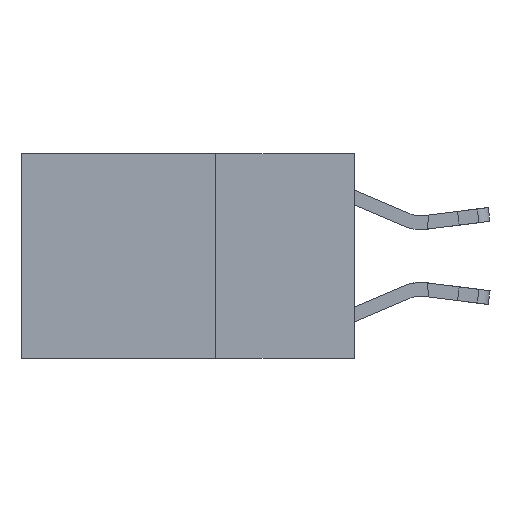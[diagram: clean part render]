
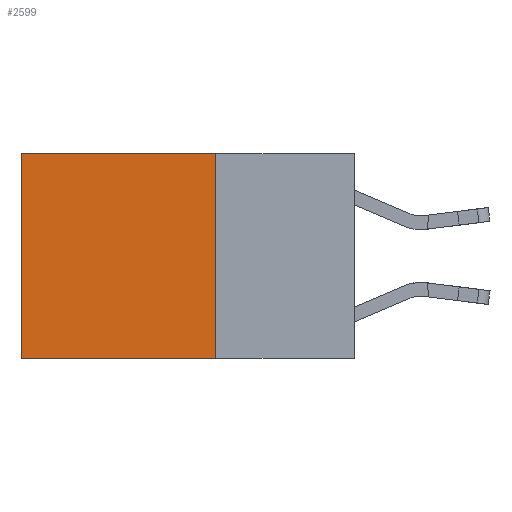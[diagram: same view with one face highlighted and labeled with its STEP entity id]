
A CAD part, left-side view. The second image highlights one B-rep face of the part: STEP entity #2599.
In plain terms, the highlighted planar face has unit normal (-1, 0, 0).
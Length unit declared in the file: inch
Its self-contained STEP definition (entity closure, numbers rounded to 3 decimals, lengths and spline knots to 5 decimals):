
#435 = VECTOR ( 'NONE', #5245, 39.37008 ) ;
#754 = LINE ( 'NONE', #13047, #18371 ) ;
#1513 = LINE ( 'NONE', #2937, #5573 ) ;
#1742 = DIRECTION ( 'NONE',  ( 0., 1., 0. ) ) ;
#2599 = ADVANCED_FACE ( 'NONE', ( #16636 ), #10279, .F. ) ;
#2937 = CARTESIAN_POINT ( 'NONE',  ( 0.2625, 0.25, 0. ) ) ;
#3076 = VERTEX_POINT ( 'NONE', #11743 ) ;
#3547 = ORIENTED_EDGE ( 'NONE', *, *, #13898, .T. ) ;
#5078 = VERTEX_POINT ( 'NONE', #19584 ) ;
#5245 = DIRECTION ( 'NONE',  ( 0., 0., -1. ) ) ;
#5573 = VECTOR ( 'NONE', #1742, 39.37008 ) ;
#5997 = ORIENTED_EDGE ( 'NONE', *, *, #12808, .F. ) ;
#6161 = EDGE_CURVE ( 'NONE', #3076, #11448, #14962, .T. ) ;
#6278 = AXIS2_PLACEMENT_3D ( 'NONE', #13685, #18794, #8661 ) ;
#7258 = ORIENTED_EDGE ( 'NONE', *, *, #6161, .F. ) ;
#7302 = EDGE_LOOP ( 'NONE', ( #21261, #7258, #5997, #3547 ) ) ;
#8661 = DIRECTION ( 'NONE',  ( 0., 0., -1. ) ) ;
#9458 = EDGE_CURVE ( 'NONE', #12452, #11448, #13536, .T. ) ;
#10279 = PLANE ( 'NONE',  #6278 ) ;
#10459 = VECTOR ( 'NONE', #15461, 39.37008 ) ;
#11448 = VERTEX_POINT ( 'NONE', #21398 ) ;
#11743 = CARTESIAN_POINT ( 'NONE',  ( 0.2625, 0.25, -0.37 ) ) ;
#12452 = VERTEX_POINT ( 'NONE', #20598 ) ;
#12808 = EDGE_CURVE ( 'NONE', #5078, #3076, #754, .T. ) ;
#13047 = CARTESIAN_POINT ( 'NONE',  ( 0.2625, 0.25, 0. ) ) ;
#13536 = LINE ( 'NONE', #17143, #435 ) ;
#13685 = CARTESIAN_POINT ( 'NONE',  ( 0.2625, 0.25, 0. ) ) ;
#13898 = EDGE_CURVE ( 'NONE', #5078, #12452, #1513, .T. ) ;
#14962 = LINE ( 'NONE', #20484, #10459 ) ;
#15461 = DIRECTION ( 'NONE',  ( 0., 1., 0. ) ) ;
#16636 = FACE_OUTER_BOUND ( 'NONE', #7302, .T. ) ;
#17143 = CARTESIAN_POINT ( 'NONE',  ( 0.2625, 0.6, 0. ) ) ;
#18173 = DIRECTION ( 'NONE',  ( 0., 0., -1. ) ) ;
#18371 = VECTOR ( 'NONE', #18173, 39.37008 ) ;
#18794 = DIRECTION ( 'NONE',  ( 1., 0., 0. ) ) ;
#19584 = CARTESIAN_POINT ( 'NONE',  ( 0.2625, 0.25, 0. ) ) ;
#20484 = CARTESIAN_POINT ( 'NONE',  ( 0.2625, 0.25, -0.37 ) ) ;
#20598 = CARTESIAN_POINT ( 'NONE',  ( 0.2625, 0.6, 0. ) ) ;
#21261 = ORIENTED_EDGE ( 'NONE', *, *, #9458, .T. ) ;
#21398 = CARTESIAN_POINT ( 'NONE',  ( 0.2625, 0.6, -0.37 ) ) ;
